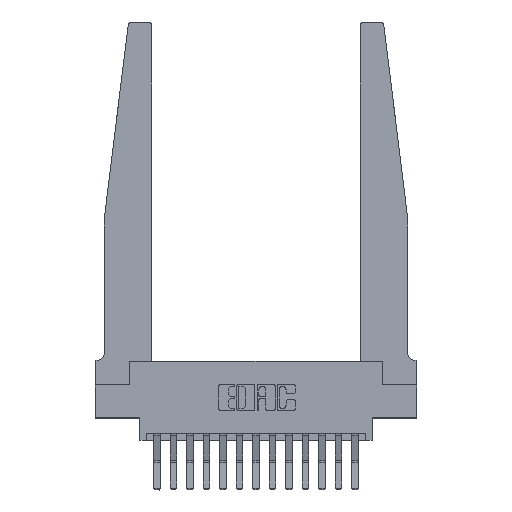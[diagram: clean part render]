
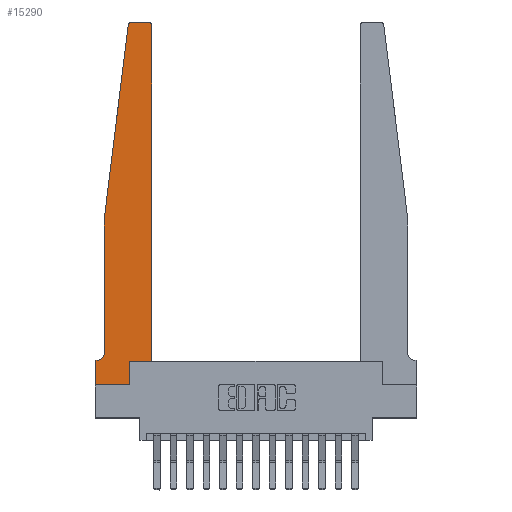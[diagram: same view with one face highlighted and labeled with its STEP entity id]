
A CAD part, top view. The second image highlights one B-rep face of the part: STEP entity #15290.
In plain terms, the highlighted planar face has unit normal (0, 0, 1).
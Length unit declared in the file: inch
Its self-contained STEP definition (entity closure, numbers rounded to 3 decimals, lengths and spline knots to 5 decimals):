
#11 = VERTEX_POINT ( 'NONE', #16328 ) ;
#394 = DIRECTION ( 'NONE',  ( 0., 0., 1. ) ) ;
#580 = FACE_OUTER_BOUND ( 'NONE', #5373, .T. ) ;
#813 = VERTEX_POINT ( 'NONE', #10931 ) ;
#925 = CARTESIAN_POINT ( 'NONE',  ( 0.27653, 2.72, 0.37 ) ) ;
#989 = CARTESIAN_POINT ( 'NONE',  ( 0.015, 0.2375, 0.37 ) ) ;
#1274 = CIRCLE ( 'NONE', #2015, 0.03 ) ;
#1309 = CARTESIAN_POINT ( 'NONE',  ( 0.065, 1.25, 0.37 ) ) ;
#1651 = CARTESIAN_POINT ( 'NONE',  ( 0.395, 2.72, 0.37 ) ) ;
#1823 = CARTESIAN_POINT ( 'NONE',  ( 0.2605, 0.18, 0.37 ) ) ;
#1853 = AXIS2_PLACEMENT_3D ( 'NONE', #989, #10408, #2357 ) ;
#1912 = VERTEX_POINT ( 'NONE', #6469 ) ;
#2015 = AXIS2_PLACEMENT_3D ( 'NONE', #925, #10344, #2301 ) ;
#2096 = EDGE_CURVE ( 'NONE', #1912, #4968, #3948, .T. ) ;
#2255 = EDGE_CURVE ( 'NONE', #9297, #11496, #6377, .T. ) ;
#2301 = DIRECTION ( 'NONE',  ( 1., 0., 0. ) ) ;
#2357 = DIRECTION ( 'NONE',  ( -1., 0., 0. ) ) ;
#2575 = EDGE_CURVE ( 'NONE', #12862, #11, #1274, .T. ) ;
#2884 = CARTESIAN_POINT ( 'NONE',  ( 0.065, 0.1875, 0.37 ) ) ;
#3019 = DIRECTION ( 'NONE',  ( 1., 0., 0. ) ) ;
#3028 = ORIENTED_EDGE ( 'NONE', *, *, #10473, .T. ) ;
#3125 = DIRECTION ( 'NONE',  ( 1., 0., 0. ) ) ;
#3186 = ORIENTED_EDGE ( 'NONE', *, *, #9279, .T. ) ;
#3948 = LINE ( 'NONE', #1309, #15151 ) ;
#3954 = VECTOR ( 'NONE', #16319, 39.37008 ) ;
#4168 = VECTOR ( 'NONE', #5234, 39.37008 ) ;
#4180 = EDGE_CURVE ( 'NONE', #4941, #813, #9424, .T. ) ;
#4646 = ORIENTED_EDGE ( 'NONE', *, *, #10372, .T. ) ;
#4731 = ORIENTED_EDGE ( 'NONE', *, *, #2096, .T. ) ;
#4941 = VERTEX_POINT ( 'NONE', #16070 ) ;
#4968 = VERTEX_POINT ( 'NONE', #6806 ) ;
#5077 = EDGE_CURVE ( 'NONE', #11496, #12862, #7115, .T. ) ;
#5160 = VECTOR ( 'NONE', #3125, 39.37008 ) ;
#5234 = DIRECTION ( 'NONE',  ( -0.122, -0.992, 0. ) ) ;
#5373 = EDGE_LOOP ( 'NONE', ( #5884, #16205, #13464, #4731, #11436, #3186, #7283, #6281, #3028, #14180, #4646, #6057 ) ) ;
#5746 = PLANE ( 'NONE',  #9017 ) ;
#5884 = ORIENTED_EDGE ( 'NONE', *, *, #5077, .T. ) ;
#6057 = ORIENTED_EDGE ( 'NONE', *, *, #2255, .T. ) ;
#6101 = VECTOR ( 'NONE', #10925, 39.37008 ) ;
#6281 = ORIENTED_EDGE ( 'NONE', *, *, #16472, .T. ) ;
#6377 = CIRCLE ( 'NONE', #15271, 0.03 ) ;
#6469 = CARTESIAN_POINT ( 'NONE',  ( 0.065, 1.25, 0.37 ) ) ;
#6745 = CIRCLE ( 'NONE', #1853, 0.05 ) ;
#6806 = CARTESIAN_POINT ( 'NONE',  ( 0.065, 0.2375, 0.37 ) ) ;
#6986 = CARTESIAN_POINT ( 'NONE',  ( 0.425, 0.18, 0.37 ) ) ;
#7049 = EDGE_CURVE ( 'NONE', #10183, #8669, #7865, .T. ) ;
#7115 = LINE ( 'NONE', #11056, #10236 ) ;
#7220 = DIRECTION ( 'NONE',  ( 1., 0., 0. ) ) ;
#7283 = ORIENTED_EDGE ( 'NONE', *, *, #4180, .T. ) ;
#7514 = LINE ( 'NONE', #14993, #3954 ) ;
#7865 = LINE ( 'NONE', #11162, #5160 ) ;
#8073 = DIRECTION ( 'NONE',  ( 0., -1., 0. ) ) ;
#8544 = VERTEX_POINT ( 'NONE', #15835 ) ;
#8669 = VERTEX_POINT ( 'NONE', #6986 ) ;
#8732 = LINE ( 'NONE', #15220, #9154 ) ;
#8970 = CARTESIAN_POINT ( 'NONE',  ( 0.395, 2.75, 0.37 ) ) ;
#8989 = EDGE_CURVE ( 'NONE', #4968, #11602, #6745, .T. ) ;
#9017 = AXIS2_PLACEMENT_3D ( 'NONE', #11118, #394, #9825 ) ;
#9154 = VECTOR ( 'NONE', #7220, 39.37008 ) ;
#9279 = EDGE_CURVE ( 'NONE', #11602, #4941, #16329, .T. ) ;
#9297 = VERTEX_POINT ( 'NONE', #12336 ) ;
#9390 = VECTOR ( 'NONE', #11242, 39.37008 ) ;
#9424 = LINE ( 'NONE', #14666, #16108 ) ;
#9825 = DIRECTION ( 'NONE',  ( 1., 0., 0. ) ) ;
#10120 = EDGE_CURVE ( 'NONE', #11, #1912, #14443, .T. ) ;
#10183 = VERTEX_POINT ( 'NONE', #14660 ) ;
#10236 = VECTOR ( 'NONE', #12397, 39.37008 ) ;
#10344 = DIRECTION ( 'NONE',  ( 0., 0., 1. ) ) ;
#10372 = EDGE_CURVE ( 'NONE', #8669, #9297, #7514, .T. ) ;
#10408 = DIRECTION ( 'NONE',  ( 0., 0., -1. ) ) ;
#10473 = EDGE_CURVE ( 'NONE', #8544, #10183, #12964, .T. ) ;
#10925 = DIRECTION ( 'NONE',  ( -1., 0., 0. ) ) ;
#10931 = CARTESIAN_POINT ( 'NONE',  ( 0., 0., 0.37 ) ) ;
#11056 = CARTESIAN_POINT ( 'NONE',  ( 0.25, 2.75, 0.37 ) ) ;
#11062 = DIRECTION ( 'NONE',  ( 0., 0., 1. ) ) ;
#11118 = CARTESIAN_POINT ( 'NONE',  ( 0., 0.1875, 0.37 ) ) ;
#11162 = CARTESIAN_POINT ( 'NONE',  ( 0.425, 0.18, 0.37 ) ) ;
#11242 = DIRECTION ( 'NONE',  ( 0., 1., 0. ) ) ;
#11436 = ORIENTED_EDGE ( 'NONE', *, *, #8989, .T. ) ;
#11496 = VERTEX_POINT ( 'NONE', #8970 ) ;
#11602 = VERTEX_POINT ( 'NONE', #11847 ) ;
#11847 = CARTESIAN_POINT ( 'NONE',  ( 0.015, 0.1875, 0.37 ) ) ;
#11967 = DIRECTION ( 'NONE',  ( 0., -1., 0. ) ) ;
#12336 = CARTESIAN_POINT ( 'NONE',  ( 0.425, 2.72, 0.37 ) ) ;
#12397 = DIRECTION ( 'NONE',  ( -1., 0., 0. ) ) ;
#12862 = VERTEX_POINT ( 'NONE', #14574 ) ;
#12964 = LINE ( 'NONE', #1823, #9390 ) ;
#13253 = CARTESIAN_POINT ( 'NONE',  ( 0.065, 1.25, 0.37 ) ) ;
#13464 = ORIENTED_EDGE ( 'NONE', *, *, #10120, .T. ) ;
#14180 = ORIENTED_EDGE ( 'NONE', *, *, #7049, .T. ) ;
#14443 = LINE ( 'NONE', #13253, #4168 ) ;
#14574 = CARTESIAN_POINT ( 'NONE',  ( 0.27653, 2.75, 0.37 ) ) ;
#14660 = CARTESIAN_POINT ( 'NONE',  ( 0.2605, 0.18, 0.37 ) ) ;
#14666 = CARTESIAN_POINT ( 'NONE',  ( 0., 0., 0.37 ) ) ;
#14993 = CARTESIAN_POINT ( 'NONE',  ( 0.425, 0.18, 0.37 ) ) ;
#15151 = VECTOR ( 'NONE', #8073, 39.37008 ) ;
#15220 = CARTESIAN_POINT ( 'NONE',  ( 0., 0., 0.37 ) ) ;
#15271 = AXIS2_PLACEMENT_3D ( 'NONE', #1651, #11062, #3019 ) ;
#15290 = ADVANCED_FACE ( 'NONE', ( #580 ), #5746, .T. ) ;
#15835 = CARTESIAN_POINT ( 'NONE',  ( 0.2605, 0., 0.37 ) ) ;
#16070 = CARTESIAN_POINT ( 'NONE',  ( 0., 0.1875, 0.37 ) ) ;
#16108 = VECTOR ( 'NONE', #11967, 39.37008 ) ;
#16205 = ORIENTED_EDGE ( 'NONE', *, *, #2575, .T. ) ;
#16319 = DIRECTION ( 'NONE',  ( 0., 1., 0. ) ) ;
#16328 = CARTESIAN_POINT ( 'NONE',  ( 0.24675, 2.72367, 0.37 ) ) ;
#16329 = LINE ( 'NONE', #2884, #6101 ) ;
#16472 = EDGE_CURVE ( 'NONE', #813, #8544, #8732, .T. ) ;
